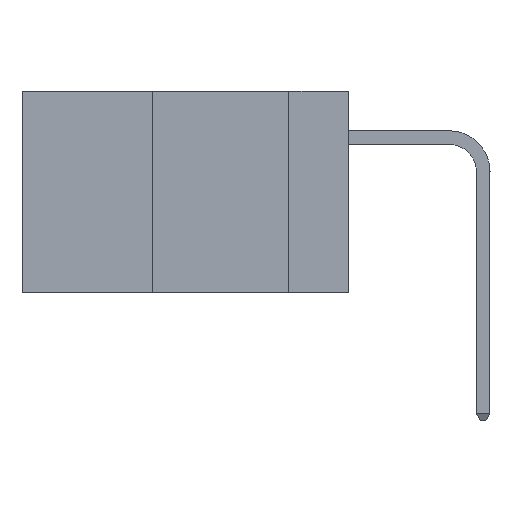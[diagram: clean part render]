
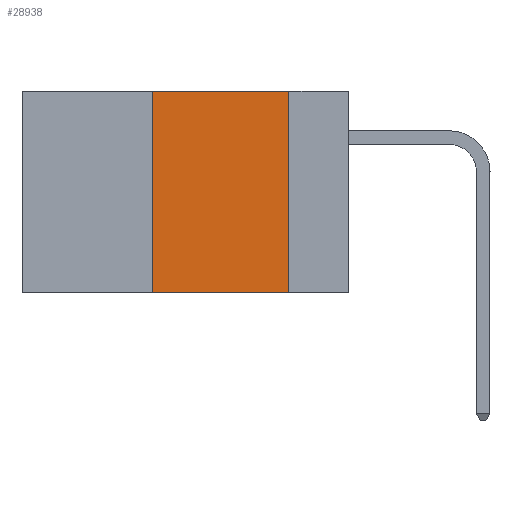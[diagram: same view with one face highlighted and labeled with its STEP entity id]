
A CAD part, left-side view. The second image highlights one B-rep face of the part: STEP entity #28938.
In plain terms, the highlighted planar face has unit normal (-1, 0, 0).
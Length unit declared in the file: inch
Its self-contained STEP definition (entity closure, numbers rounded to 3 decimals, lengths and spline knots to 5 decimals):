
#1643 = ORIENTED_EDGE ( 'NONE', *, *, #26683, .F. ) ;
#2147 = CARTESIAN_POINT ( 'NONE',  ( 0., 0.6, 0. ) ) ;
#3634 = PLANE ( 'NONE',  #33060 ) ;
#5190 = VECTOR ( 'NONE', #41522, 39.37008 ) ;
#5500 = ORIENTED_EDGE ( 'NONE', *, *, #17336, .F. ) ;
#6456 = FACE_OUTER_BOUND ( 'NONE', #40511, .T. ) ;
#7143 = CARTESIAN_POINT ( 'NONE',  ( 0., 0.6, 0. ) ) ;
#8230 = LINE ( 'NONE', #35081, #29614 ) ;
#8341 = LINE ( 'NONE', #43626, #24770 ) ;
#9363 = VERTEX_POINT ( 'NONE', #10361 ) ;
#10229 = CARTESIAN_POINT ( 'NONE',  ( 0., 0.11, 0. ) ) ;
#10361 = CARTESIAN_POINT ( 'NONE',  ( 0., 0.36, 0. ) ) ;
#10429 = ORIENTED_EDGE ( 'NONE', *, *, #21843, .F. ) ;
#10723 = DIRECTION ( 'NONE',  ( 0., 0., -1. ) ) ;
#11591 = CARTESIAN_POINT ( 'NONE',  ( 0., 0.11, -0.37 ) ) ;
#15951 = LINE ( 'NONE', #2147, #24153 ) ;
#17336 = EDGE_CURVE ( 'NONE', #22579, #34589, #8341, .T. ) ;
#19046 = EDGE_CURVE ( 'NONE', #32782, #34589, #8230, .T. ) ;
#21843 = EDGE_CURVE ( 'NONE', #32782, #9363, #37540, .T. ) ;
#22579 = VERTEX_POINT ( 'NONE', #10229 ) ;
#23660 = CARTESIAN_POINT ( 'NONE',  ( 0., 0.36, -0.37 ) ) ;
#24153 = VECTOR ( 'NONE', #33571, 39.37008 ) ;
#24770 = VECTOR ( 'NONE', #36463, 39.37008 ) ;
#26683 = EDGE_CURVE ( 'NONE', #9363, #22579, #15951, .T. ) ;
#28938 = ADVANCED_FACE ( 'NONE', ( #6456 ), #3634, .F. ) ;
#29614 = VECTOR ( 'NONE', #32008, 39.37008 ) ;
#31684 = DIRECTION ( 'NONE',  ( 1., 0., 0. ) ) ;
#32008 = DIRECTION ( 'NONE',  ( 0., -1., 0. ) ) ;
#32782 = VERTEX_POINT ( 'NONE', #23660 ) ;
#33060 = AXIS2_PLACEMENT_3D ( 'NONE', #7143, #31684, #10723 ) ;
#33571 = DIRECTION ( 'NONE',  ( 0., -1., 0. ) ) ;
#34589 = VERTEX_POINT ( 'NONE', #11591 ) ;
#34633 = CARTESIAN_POINT ( 'NONE',  ( 0., 0.36, 0. ) ) ;
#35081 = CARTESIAN_POINT ( 'NONE',  ( 0., 0.6, -0.37 ) ) ;
#36463 = DIRECTION ( 'NONE',  ( 0., 0., -1. ) ) ;
#37540 = LINE ( 'NONE', #34633, #5190 ) ;
#38306 = ORIENTED_EDGE ( 'NONE', *, *, #19046, .T. ) ;
#40511 = EDGE_LOOP ( 'NONE', ( #5500, #1643, #10429, #38306 ) ) ;
#41522 = DIRECTION ( 'NONE',  ( 0., 0., 1. ) ) ;
#43626 = CARTESIAN_POINT ( 'NONE',  ( 0., 0.11, 0. ) ) ;
